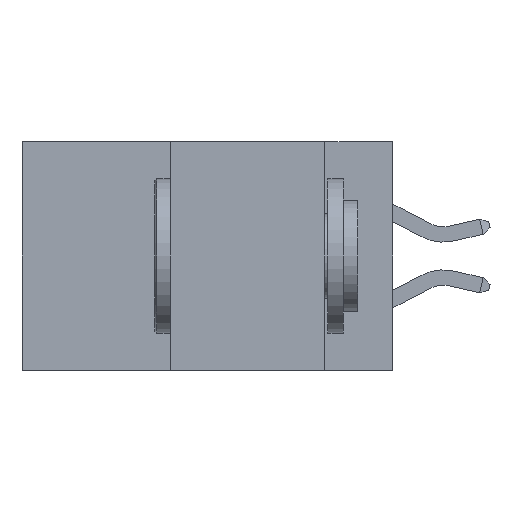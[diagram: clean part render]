
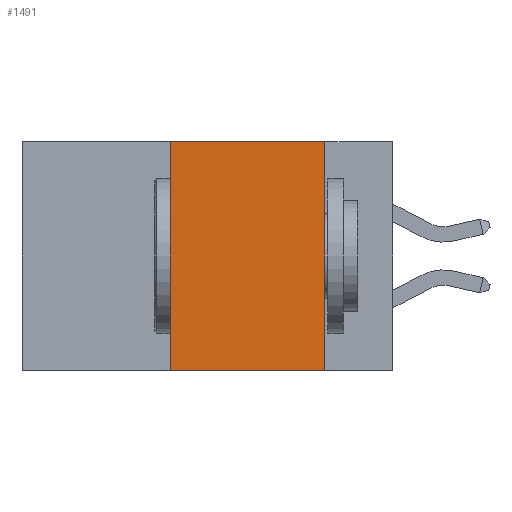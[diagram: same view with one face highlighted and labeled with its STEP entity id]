
A CAD part, left-side view. The second image highlights one B-rep face of the part: STEP entity #1491.
In plain terms, the highlighted planar face has unit normal (-1, 0, 0).
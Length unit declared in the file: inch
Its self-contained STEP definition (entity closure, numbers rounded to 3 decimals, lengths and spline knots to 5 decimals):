
#1465 = ORIENTED_EDGE ( 'NONE', *, *, #11635, .T. ) ;
#1491 = ADVANCED_FACE ( 'NONE', ( #10039 ), #12198, .F. ) ;
#1799 = VERTEX_POINT ( 'NONE', #32650 ) ;
#2374 = VERTEX_POINT ( 'NONE', #24633 ) ;
#3185 = VECTOR ( 'NONE', #3958, 39.37008 ) ;
#3529 = DIRECTION ( 'NONE',  ( 0., 0., 1. ) ) ;
#3958 = DIRECTION ( 'NONE',  ( 0., -1., 0. ) ) ;
#6318 = ORIENTED_EDGE ( 'NONE', *, *, #19326, .F. ) ;
#6723 = VERTEX_POINT ( 'NONE', #13913 ) ;
#6732 = AXIS2_PLACEMENT_3D ( 'NONE', #11724, #11444, #11362 ) ;
#8862 = VECTOR ( 'NONE', #31595, 39.37008 ) ;
#9689 = EDGE_CURVE ( 'NONE', #2374, #31916, #15374, .T. ) ;
#10039 = FACE_OUTER_BOUND ( 'NONE', #32560, .T. ) ;
#11362 = DIRECTION ( 'NONE',  ( 0., 0., -1. ) ) ;
#11444 = DIRECTION ( 'NONE',  ( 1., 0., 0. ) ) ;
#11635 = EDGE_CURVE ( 'NONE', #6723, #1799, #18648, .T. ) ;
#11724 = CARTESIAN_POINT ( 'NONE',  ( 0., 0.6, 0. ) ) ;
#12198 = PLANE ( 'NONE',  #6732 ) ;
#12461 = CARTESIAN_POINT ( 'NONE',  ( 0., 0.6, 0. ) ) ;
#13913 = CARTESIAN_POINT ( 'NONE',  ( 0., 0.36, -0.37 ) ) ;
#14496 = ORIENTED_EDGE ( 'NONE', *, *, #31020, .F. ) ;
#14521 = VECTOR ( 'NONE', #25994, 39.37008 ) ;
#15374 = LINE ( 'NONE', #12461, #14521 ) ;
#17235 = CARTESIAN_POINT ( 'NONE',  ( 0., 0.36, 0. ) ) ;
#18648 = LINE ( 'NONE', #28213, #3185 ) ;
#19326 = EDGE_CURVE ( 'NONE', #31916, #1799, #30377, .T. ) ;
#23929 = LINE ( 'NONE', #17235, #30219 ) ;
#24633 = CARTESIAN_POINT ( 'NONE',  ( 0., 0.36, 0. ) ) ;
#25994 = DIRECTION ( 'NONE',  ( 0., -1., 0. ) ) ;
#28213 = CARTESIAN_POINT ( 'NONE',  ( 0., 0.6, -0.37 ) ) ;
#28757 = ORIENTED_EDGE ( 'NONE', *, *, #9689, .F. ) ;
#30219 = VECTOR ( 'NONE', #3529, 39.37008 ) ;
#30377 = LINE ( 'NONE', #34279, #8862 ) ;
#31020 = EDGE_CURVE ( 'NONE', #6723, #2374, #23929, .T. ) ;
#31394 = CARTESIAN_POINT ( 'NONE',  ( 0., 0.11, 0. ) ) ;
#31595 = DIRECTION ( 'NONE',  ( 0., 0., -1. ) ) ;
#31916 = VERTEX_POINT ( 'NONE', #31394 ) ;
#32560 = EDGE_LOOP ( 'NONE', ( #6318, #28757, #14496, #1465 ) ) ;
#32650 = CARTESIAN_POINT ( 'NONE',  ( 0., 0.11, -0.37 ) ) ;
#34279 = CARTESIAN_POINT ( 'NONE',  ( 0., 0.11, 0. ) ) ;
